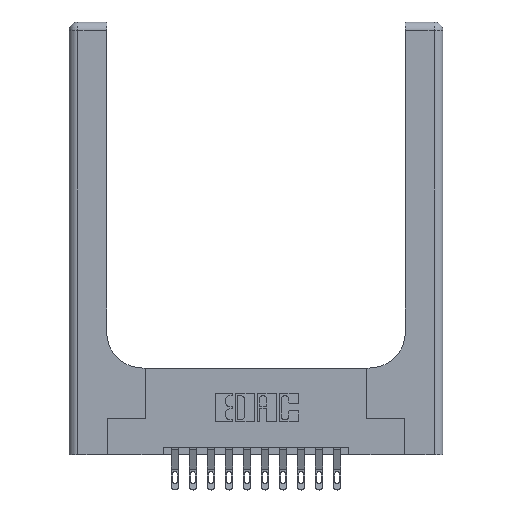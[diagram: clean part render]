
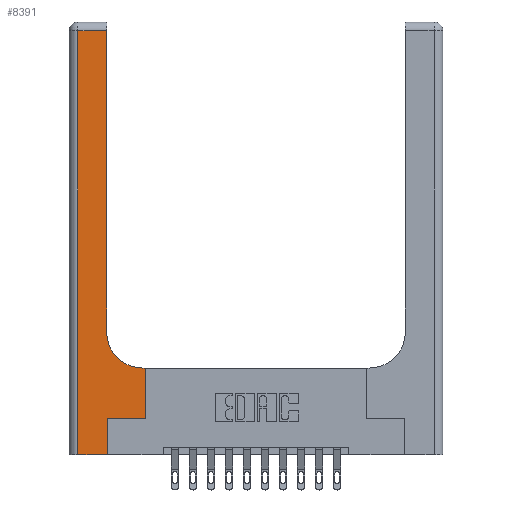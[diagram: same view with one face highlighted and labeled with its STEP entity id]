
A CAD part, top view. The second image highlights one B-rep face of the part: STEP entity #8391.
In plain terms, the highlighted planar face has unit normal (0, 0, 1).
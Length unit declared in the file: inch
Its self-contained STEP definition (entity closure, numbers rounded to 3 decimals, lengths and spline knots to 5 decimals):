
#2 = CARTESIAN_POINT ( 'NONE',  ( 0.265, 0.25, 0.37 ) ) ;
#31 = CARTESIAN_POINT ( 'NONE',  ( 0.06, 2.94, 0.37 ) ) ;
#863 = AXIS2_PLACEMENT_3D ( 'NONE', #12336, #7331, #14803 ) ;
#910 = CARTESIAN_POINT ( 'NONE',  ( 0.265, 0.25, 0.37 ) ) ;
#1108 = CARTESIAN_POINT ( 'NONE',  ( 0.528, 0.25, 0.37 ) ) ;
#1150 = DIRECTION ( 'NONE',  ( 0., 1., 0. ) ) ;
#1252 = DIRECTION ( 'NONE',  ( 1., 0., 0. ) ) ;
#1727 = CARTESIAN_POINT ( 'NONE',  ( 0.06, 0., 0.37 ) ) ;
#1936 = VERTEX_POINT ( 'NONE', #3900 ) ;
#2139 = ORIENTED_EDGE ( 'NONE', *, *, #8625, .T. ) ;
#2486 = ORIENTED_EDGE ( 'NONE', *, *, #8193, .T. ) ;
#2885 = ORIENTED_EDGE ( 'NONE', *, *, #13560, .T. ) ;
#3100 = LINE ( 'NONE', #8287, #13579 ) ;
#3900 = CARTESIAN_POINT ( 'NONE',  ( 0.26, 0.85, 0.37 ) ) ;
#3970 = DIRECTION ( 'NONE',  ( 0., 1., 0. ) ) ;
#4073 = CARTESIAN_POINT ( 'NONE',  ( 0.265, 0., 0.37 ) ) ;
#5070 = LINE ( 'NONE', #15328, #12256 ) ;
#5136 = VECTOR ( 'NONE', #11604, 39.37008 ) ;
#5347 = DIRECTION ( 'NONE',  ( 0., 0., -1. ) ) ;
#5442 = ORIENTED_EDGE ( 'NONE', *, *, #10835, .T. ) ;
#5595 = CARTESIAN_POINT ( 'NONE',  ( 0.26, 2.94, 0.37 ) ) ;
#5724 = ORIENTED_EDGE ( 'NONE', *, *, #11889, .T. ) ;
#6109 = DIRECTION ( 'NONE',  ( 1., 0., 0. ) ) ;
#6110 = VERTEX_POINT ( 'NONE', #12521 ) ;
#6216 = ORIENTED_EDGE ( 'NONE', *, *, #10616, .T. ) ;
#6269 = LINE ( 'NONE', #7804, #11186 ) ;
#6768 = EDGE_LOOP ( 'NONE', ( #5724, #2885, #2486, #5442, #12084, #6216, #15320, #2139, #13123 ) ) ;
#7224 = VECTOR ( 'NONE', #6109, 39.37008 ) ;
#7331 = DIRECTION ( 'NONE',  ( 0., 0., -1. ) ) ;
#7371 = LINE ( 'NONE', #12539, #8241 ) ;
#7804 = CARTESIAN_POINT ( 'NONE',  ( 0., 0., 0.37 ) ) ;
#7868 = VERTEX_POINT ( 'NONE', #5595 ) ;
#8076 = FACE_OUTER_BOUND ( 'NONE', #6768, .T. ) ;
#8126 = VERTEX_POINT ( 'NONE', #1727 ) ;
#8193 = EDGE_CURVE ( 'NONE', #11933, #8126, #3100, .T. ) ;
#8241 = VECTOR ( 'NONE', #15331, 39.37008 ) ;
#8287 = CARTESIAN_POINT ( 'NONE',  ( 0.06, 3., 0.37 ) ) ;
#8391 = ADVANCED_FACE ( 'NONE', ( #8076 ), #13247, .F. ) ;
#8625 = EDGE_CURVE ( 'NONE', #6110, #14252, #15404, .T. ) ;
#8659 = LINE ( 'NONE', #910, #7224 ) ;
#8985 = CARTESIAN_POINT ( 'NONE',  ( 0.26, 0.6, 0.37 ) ) ;
#9298 = CIRCLE ( 'NONE', #863, 0.25 ) ;
#10616 = EDGE_CURVE ( 'NONE', #15980, #12691, #8659, .T. ) ;
#10835 = EDGE_CURVE ( 'NONE', #8126, #14538, #6269, .T. ) ;
#11005 = VECTOR ( 'NONE', #12530, 39.37008 ) ;
#11169 = LINE ( 'NONE', #16333, #11005 ) ;
#11186 = VECTOR ( 'NONE', #1252, 39.37008 ) ;
#11604 = DIRECTION ( 'NONE',  ( -1., 0., 0. ) ) ;
#11889 = EDGE_CURVE ( 'NONE', #1936, #7868, #5070, .T. ) ;
#11933 = VERTEX_POINT ( 'NONE', #31 ) ;
#11939 = EDGE_CURVE ( 'NONE', #12691, #6110, #14071, .T. ) ;
#12084 = ORIENTED_EDGE ( 'NONE', *, *, #16653, .T. ) ;
#12256 = VECTOR ( 'NONE', #3970, 39.37008 ) ;
#12336 = CARTESIAN_POINT ( 'NONE',  ( 0.51, 0.85, 0.37 ) ) ;
#12501 = EDGE_CURVE ( 'NONE', #14252, #1936, #9298, .T. ) ;
#12518 = VECTOR ( 'NONE', #1150, 39.37008 ) ;
#12521 = CARTESIAN_POINT ( 'NONE',  ( 0.528, 0.6, 0.37 ) ) ;
#12530 = DIRECTION ( 'NONE',  ( 0., 1., 0. ) ) ;
#12539 = CARTESIAN_POINT ( 'NONE',  ( 0., 2.94, 0.37 ) ) ;
#12691 = VERTEX_POINT ( 'NONE', #1108 ) ;
#12779 = CARTESIAN_POINT ( 'NONE',  ( 0.528, 0.25, 0.37 ) ) ;
#13123 = ORIENTED_EDGE ( 'NONE', *, *, #12501, .T. ) ;
#13247 = PLANE ( 'NONE',  #14089 ) ;
#13421 = DIRECTION ( 'NONE',  ( -1., 0., 0. ) ) ;
#13463 = DIRECTION ( 'NONE',  ( 0., -1., 0. ) ) ;
#13524 = CARTESIAN_POINT ( 'NONE',  ( 0.51, 0.6, 0.37 ) ) ;
#13560 = EDGE_CURVE ( 'NONE', #7868, #11933, #7371, .T. ) ;
#13579 = VECTOR ( 'NONE', #13463, 39.37008 ) ;
#14071 = LINE ( 'NONE', #12779, #12518 ) ;
#14089 = AXIS2_PLACEMENT_3D ( 'NONE', #15677, #5347, #13421 ) ;
#14252 = VERTEX_POINT ( 'NONE', #13524 ) ;
#14538 = VERTEX_POINT ( 'NONE', #4073 ) ;
#14803 = DIRECTION ( 'NONE',  ( 1., 0., 0. ) ) ;
#15320 = ORIENTED_EDGE ( 'NONE', *, *, #11939, .T. ) ;
#15328 = CARTESIAN_POINT ( 'NONE',  ( 0.26, 3., 0.37 ) ) ;
#15331 = DIRECTION ( 'NONE',  ( -1., 0., 0. ) ) ;
#15404 = LINE ( 'NONE', #8985, #5136 ) ;
#15677 = CARTESIAN_POINT ( 'NONE',  ( 0., 3., 0.37 ) ) ;
#15980 = VERTEX_POINT ( 'NONE', #2 ) ;
#16333 = CARTESIAN_POINT ( 'NONE',  ( 0.265, 0., 0.37 ) ) ;
#16653 = EDGE_CURVE ( 'NONE', #14538, #15980, #11169, .T. ) ;
